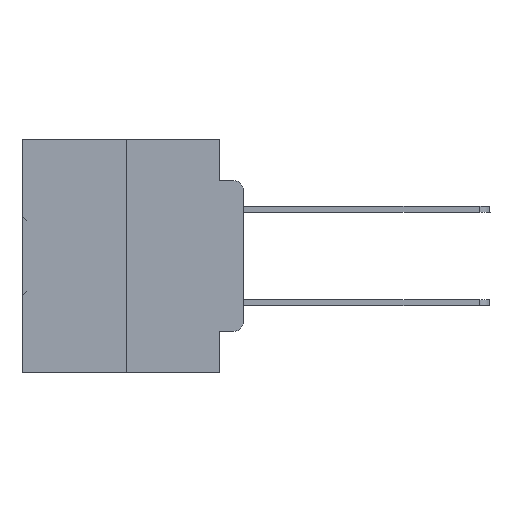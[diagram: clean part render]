
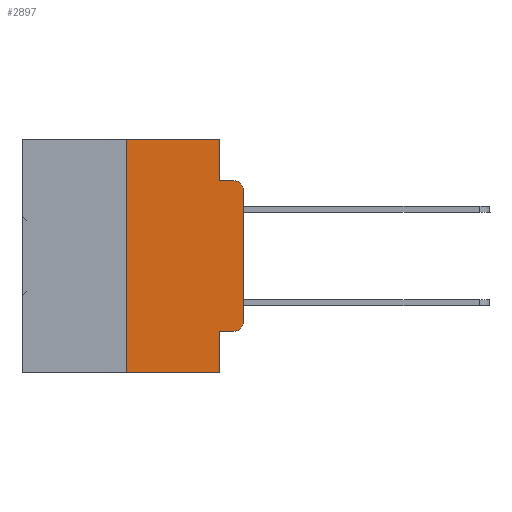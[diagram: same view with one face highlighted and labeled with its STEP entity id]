
A CAD part, left-side view. The second image highlights one B-rep face of the part: STEP entity #2897.
In plain terms, the highlighted planar face has unit normal (-1, 0, 0).
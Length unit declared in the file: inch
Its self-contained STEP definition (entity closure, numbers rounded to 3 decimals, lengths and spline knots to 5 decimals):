
#134 = ORIENTED_EDGE ( 'NONE', *, *, #27759, .T. ) ;
#505 = CARTESIAN_POINT ( 'NONE',  ( 0., 0.051, 0. ) ) ;
#605 = VERTEX_POINT ( 'NONE', #17652 ) ;
#698 = LINE ( 'NONE', #5836, #13226 ) ;
#1250 = EDGE_CURVE ( 'NONE', #8806, #32176, #698, .T. ) ;
#2719 = DIRECTION ( 'NONE',  ( 0., 0., 1. ) ) ;
#2897 = ADVANCED_FACE ( 'NONE', ( #37603 ), #13692, .F. ) ;
#3296 = VECTOR ( 'NONE', #31508, 39.37008 ) ;
#3575 = VECTOR ( 'NONE', #20974, 39.37008 ) ;
#4130 = ORIENTED_EDGE ( 'NONE', *, *, #1250, .F. ) ;
#4252 = EDGE_CURVE ( 'NONE', #23312, #24308, #15551, .T. ) ;
#4740 = CARTESIAN_POINT ( 'NONE',  ( 0., 0.473, -0.5 ) ) ;
#5287 = DIRECTION ( 'NONE',  ( 0., 0., -1. ) ) ;
#5508 = EDGE_CURVE ( 'NONE', #6010, #31991, #11713, .T. ) ;
#5836 = CARTESIAN_POINT ( 'NONE',  ( 0., 0.25, 0. ) ) ;
#6010 = VERTEX_POINT ( 'NONE', #18474 ) ;
#6598 = CARTESIAN_POINT ( 'NONE',  ( 0., 0.02, -0.4115 ) ) ;
#7737 = CARTESIAN_POINT ( 'NONE',  ( 0., 0.051, -0.5 ) ) ;
#7863 = LINE ( 'NONE', #36681, #25114 ) ;
#8806 = VERTEX_POINT ( 'NONE', #32609 ) ;
#8876 = LINE ( 'NONE', #31381, #3296 ) ;
#9380 = VECTOR ( 'NONE', #17864, 39.37008 ) ;
#9517 = EDGE_CURVE ( 'NONE', #14911, #605, #8876, .T. ) ;
#9603 = CARTESIAN_POINT ( 'NONE',  ( 0., 0.051, 0. ) ) ;
#10232 = CARTESIAN_POINT ( 'NONE',  ( 0., 0.25, 0. ) ) ;
#11713 = LINE ( 'NONE', #23640, #9380 ) ;
#11725 = AXIS2_PLACEMENT_3D ( 'NONE', #16804, #37615, #11792 ) ;
#11792 = DIRECTION ( 'NONE',  ( 0., 0., -1. ) ) ;
#13226 = VECTOR ( 'NONE', #2719, 39.37008 ) ;
#13653 = ORIENTED_EDGE ( 'NONE', *, *, #27975, .F. ) ;
#13692 = PLANE ( 'NONE',  #28334 ) ;
#14682 = ORIENTED_EDGE ( 'NONE', *, *, #38082, .F. ) ;
#14911 = VERTEX_POINT ( 'NONE', #18473 ) ;
#15551 = LINE ( 'NONE', #26108, #24460 ) ;
#16328 = ORIENTED_EDGE ( 'NONE', *, *, #5508, .T. ) ;
#16738 = DIRECTION ( 'NONE',  ( 1., 0., 0. ) ) ;
#16804 = CARTESIAN_POINT ( 'NONE',  ( 0., 0.02, -0.1085 ) ) ;
#17028 = ORIENTED_EDGE ( 'NONE', *, *, #9517, .F. ) ;
#17133 = LINE ( 'NONE', #505, #3575 ) ;
#17652 = CARTESIAN_POINT ( 'NONE',  ( 0., 0.02, -0.0885 ) ) ;
#17827 = AXIS2_PLACEMENT_3D ( 'NONE', #23158, #34459, #5287 ) ;
#17864 = DIRECTION ( 'NONE',  ( 0., 0., 1. ) ) ;
#18473 = CARTESIAN_POINT ( 'NONE',  ( 0., 0.051, -0.0885 ) ) ;
#18474 = CARTESIAN_POINT ( 'NONE',  ( 0., 0., -0.3915 ) ) ;
#18809 = VERTEX_POINT ( 'NONE', #9603 ) ;
#20974 = DIRECTION ( 'NONE',  ( 0., 0., -1. ) ) ;
#22967 = LINE ( 'NONE', #26983, #31306 ) ;
#23158 = CARTESIAN_POINT ( 'NONE',  ( 0., 0.02, -0.3915 ) ) ;
#23312 = VERTEX_POINT ( 'NONE', #37435 ) ;
#23640 = CARTESIAN_POINT ( 'NONE',  ( 0., 0., 0. ) ) ;
#24250 = DIRECTION ( 'NONE',  ( 0., -1., 0. ) ) ;
#24308 = VERTEX_POINT ( 'NONE', #6598 ) ;
#24460 = VECTOR ( 'NONE', #29587, 39.37008 ) ;
#25114 = VECTOR ( 'NONE', #30065, 39.37008 ) ;
#25649 = ORIENTED_EDGE ( 'NONE', *, *, #4252, .T. ) ;
#26108 = CARTESIAN_POINT ( 'NONE',  ( 0., 0.051, -0.4115 ) ) ;
#26838 = EDGE_LOOP ( 'NONE', ( #16328, #134, #17028, #29551, #14682, #4130, #30669, #13653, #25649, #28198 ) ) ;
#26976 = EDGE_CURVE ( 'NONE', #8806, #31504, #36735, .T. ) ;
#26983 = CARTESIAN_POINT ( 'NONE',  ( 0., 0.473, 0. ) ) ;
#27759 = EDGE_CURVE ( 'NONE', #31991, #605, #28809, .T. ) ;
#27975 = EDGE_CURVE ( 'NONE', #23312, #31504, #17133, .T. ) ;
#28198 = ORIENTED_EDGE ( 'NONE', *, *, #29867, .T. ) ;
#28334 = AXIS2_PLACEMENT_3D ( 'NONE', #34578, #16738, #28725 ) ;
#28725 = DIRECTION ( 'NONE',  ( 0., 0., -1. ) ) ;
#28809 = CIRCLE ( 'NONE', #11725, 0.02 ) ;
#28839 = DIRECTION ( 'NONE',  ( 0., -1., 0. ) ) ;
#29551 = ORIENTED_EDGE ( 'NONE', *, *, #36336, .F. ) ;
#29587 = DIRECTION ( 'NONE',  ( 0., -1., 0. ) ) ;
#29867 = EDGE_CURVE ( 'NONE', #24308, #6010, #34928, .T. ) ;
#30065 = DIRECTION ( 'NONE',  ( 0., 0., -1. ) ) ;
#30669 = ORIENTED_EDGE ( 'NONE', *, *, #26976, .T. ) ;
#30987 = CARTESIAN_POINT ( 'NONE',  ( 0., 0., -0.1085 ) ) ;
#31306 = VECTOR ( 'NONE', #24250, 39.37008 ) ;
#31381 = CARTESIAN_POINT ( 'NONE',  ( 0., 0.051, -0.0885 ) ) ;
#31504 = VERTEX_POINT ( 'NONE', #7737 ) ;
#31508 = DIRECTION ( 'NONE',  ( 0., -1., 0. ) ) ;
#31991 = VERTEX_POINT ( 'NONE', #30987 ) ;
#32157 = VECTOR ( 'NONE', #28839, 39.37008 ) ;
#32176 = VERTEX_POINT ( 'NONE', #10232 ) ;
#32609 = CARTESIAN_POINT ( 'NONE',  ( 0., 0.25, -0.5 ) ) ;
#34459 = DIRECTION ( 'NONE',  ( -1., 0., 0. ) ) ;
#34578 = CARTESIAN_POINT ( 'NONE',  ( 0., 0.473, 0. ) ) ;
#34928 = CIRCLE ( 'NONE', #17827, 0.02 ) ;
#36336 = EDGE_CURVE ( 'NONE', #18809, #14911, #7863, .T. ) ;
#36681 = CARTESIAN_POINT ( 'NONE',  ( 0., 0.051, 0. ) ) ;
#36735 = LINE ( 'NONE', #4740, #32157 ) ;
#37435 = CARTESIAN_POINT ( 'NONE',  ( 0., 0.051, -0.4115 ) ) ;
#37603 = FACE_OUTER_BOUND ( 'NONE', #26838, .T. ) ;
#37615 = DIRECTION ( 'NONE',  ( -1., 0., 0. ) ) ;
#38082 = EDGE_CURVE ( 'NONE', #32176, #18809, #22967, .T. ) ;
